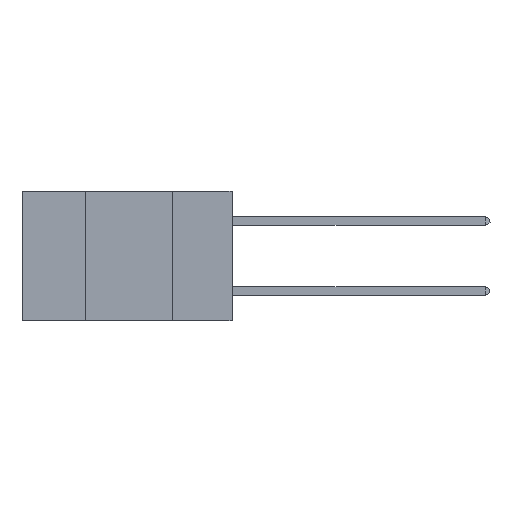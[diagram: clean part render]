
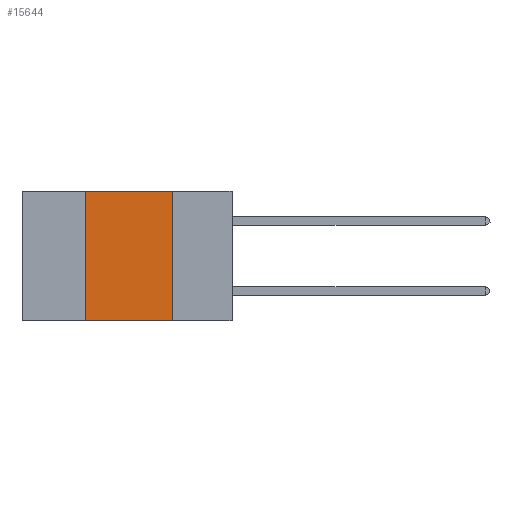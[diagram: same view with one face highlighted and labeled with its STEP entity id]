
A CAD part, left-side view. The second image highlights one B-rep face of the part: STEP entity #15644.
In plain terms, the highlighted planar face has unit normal (-1, 0, 0).
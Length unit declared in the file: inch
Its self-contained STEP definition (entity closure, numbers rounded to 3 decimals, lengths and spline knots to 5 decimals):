
#378 = ORIENTED_EDGE ( 'NONE', *, *, #11462, .F. ) ;
#1462 = VERTEX_POINT ( 'NONE', #1463 ) ;
#1463 = CARTESIAN_POINT ( 'NONE',  ( 0., 0.42, 0. ) ) ;
#1761 = DIRECTION ( 'NONE',  ( 0., 0., -1. ) ) ;
#2312 = PLANE ( 'NONE',  #15319 ) ;
#3450 = CARTESIAN_POINT ( 'NONE',  ( 0., 0.17, 0. ) ) ;
#4300 = LINE ( 'NONE', #15374, #13272 ) ;
#5311 = EDGE_CURVE ( 'NONE', #21081, #9023, #17622, .T. ) ;
#5431 = EDGE_CURVE ( 'NONE', #15812, #9023, #10102, .T. ) ;
#6270 = CARTESIAN_POINT ( 'NONE',  ( 0., 0.17, -0.37 ) ) ;
#6675 = VECTOR ( 'NONE', #20591, 39.37008 ) ;
#8129 = CARTESIAN_POINT ( 'NONE',  ( 0., 0.6, 0. ) ) ;
#9023 = VERTEX_POINT ( 'NONE', #6270 ) ;
#10102 = LINE ( 'NONE', #20710, #16220 ) ;
#11462 = EDGE_CURVE ( 'NONE', #15812, #1462, #4300, .T. ) ;
#12032 = ORIENTED_EDGE ( 'NONE', *, *, #17374, .F. ) ;
#12893 = FACE_OUTER_BOUND ( 'NONE', #16047, .T. ) ;
#12897 = VECTOR ( 'NONE', #17526, 39.37008 ) ;
#13272 = VECTOR ( 'NONE', #17158, 39.37008 ) ;
#13674 = ORIENTED_EDGE ( 'NONE', *, *, #5431, .T. ) ;
#14289 = CARTESIAN_POINT ( 'NONE',  ( 0., 0.17, 0. ) ) ;
#14320 = DIRECTION ( 'NONE',  ( 1., 0., 0. ) ) ;
#14916 = CARTESIAN_POINT ( 'NONE',  ( 0., 0.6, 0. ) ) ;
#15319 = AXIS2_PLACEMENT_3D ( 'NONE', #14916, #14320, #1761 ) ;
#15374 = CARTESIAN_POINT ( 'NONE',  ( 0., 0.42, 0. ) ) ;
#15644 = ADVANCED_FACE ( 'NONE', ( #12893 ), #2312, .F. ) ;
#15796 = ORIENTED_EDGE ( 'NONE', *, *, #5311, .F. ) ;
#15812 = VERTEX_POINT ( 'NONE', #17090 ) ;
#16047 = EDGE_LOOP ( 'NONE', ( #15796, #12032, #378, #13674 ) ) ;
#16179 = LINE ( 'NONE', #8129, #6675 ) ;
#16220 = VECTOR ( 'NONE', #22512, 39.37008 ) ;
#17090 = CARTESIAN_POINT ( 'NONE',  ( 0., 0.42, -0.37 ) ) ;
#17158 = DIRECTION ( 'NONE',  ( 0., 0., 1. ) ) ;
#17374 = EDGE_CURVE ( 'NONE', #1462, #21081, #16179, .T. ) ;
#17526 = DIRECTION ( 'NONE',  ( 0., 0., -1. ) ) ;
#17622 = LINE ( 'NONE', #3450, #12897 ) ;
#20591 = DIRECTION ( 'NONE',  ( 0., -1., 0. ) ) ;
#20710 = CARTESIAN_POINT ( 'NONE',  ( 0., 0.6, -0.37 ) ) ;
#21081 = VERTEX_POINT ( 'NONE', #14289 ) ;
#22512 = DIRECTION ( 'NONE',  ( 0., -1., 0. ) ) ;
